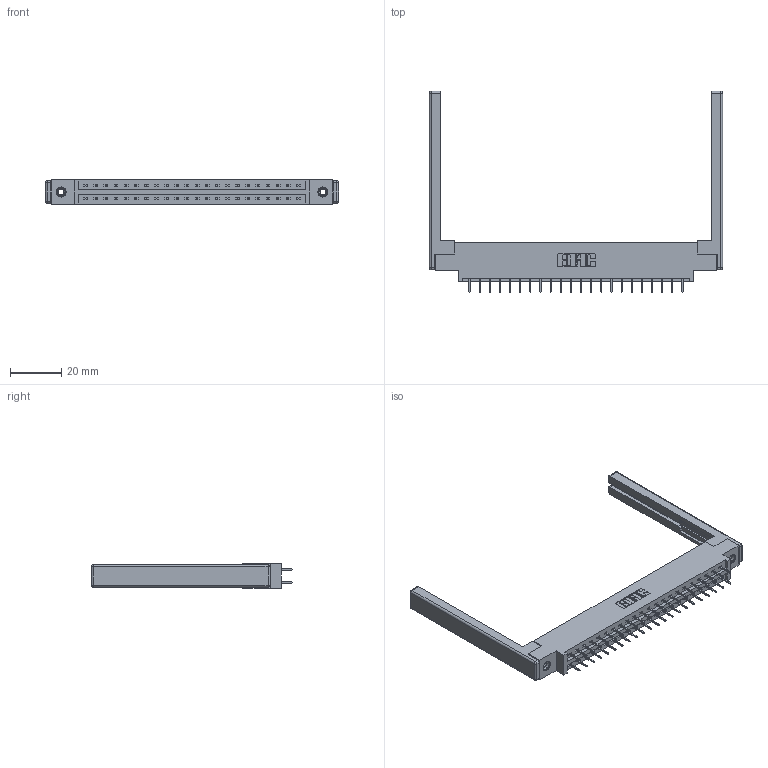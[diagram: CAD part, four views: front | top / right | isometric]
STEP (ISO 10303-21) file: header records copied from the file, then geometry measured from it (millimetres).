
FILE_DESCRIPTION (( 'STEP AP203' ), '1' );
FILE_NAME ('387-044-524-868.STEP', '2019-10-18T05:35:02', ( '' ), ( '' ), 'SwSTEP 2.0', 'SolidWorks 2016', '' );
FILE_SCHEMA (( 'CONFIG_CONTROL_DESIGN' ));
Length unit declared in the file: inch
Products named in the file (5): 345-292-001_345-293-124; 345-250-001_345-250-001-102; 337 Part_0.170 Offset - 0.156 Dia-TI; 387-044-524-868; 307-220-068
Assembly tree (49 placements, depth 2):
  387-044-524-868
    337 Part_0.170 Offset - 0.156 Dia-TI
    345-292-001_345-293-124  x44
    345-250-001_345-250-001-102  x2
    307-220-068  x2
Bounding box: 114.6 x 78.75 x 9.4 mm (x, y, z)
Volume: 16012.4 mm3; surface area: 16886.8 mm2
Topology: 49 solids, 49 shells, 2824 faces, 7973 edges, 5118 vertices
Faces by surface type: plane 2098, cylinder 702, cone 12, sphere 8, torus 4
Entity records: 22610 total; most frequent: CARTESIAN_POINT 3791, ORIENTED_EDGE 3716, DIRECTION 3332, EDGE_CURVE 1858, LINE 1684, VECTOR 1684, VERTEX_POINT 1226, AXIS2_PLACEMENT_3D 824
